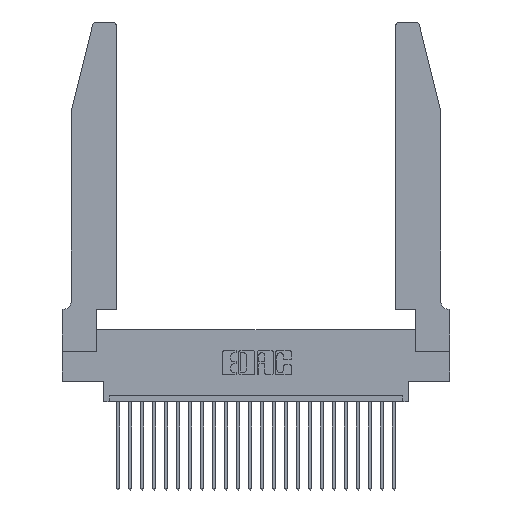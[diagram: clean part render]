
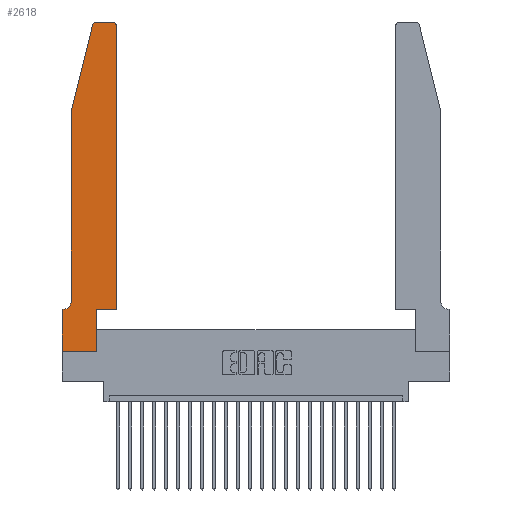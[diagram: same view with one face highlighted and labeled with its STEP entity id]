
A CAD part, top view. The second image highlights one B-rep face of the part: STEP entity #2618.
In plain terms, the highlighted planar face has unit normal (0, 0, 1).
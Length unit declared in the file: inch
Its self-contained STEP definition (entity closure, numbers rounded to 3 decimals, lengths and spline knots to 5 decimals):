
#230 = VERTEX_POINT ( 'NONE', #23160 ) ;
#433 = DIRECTION ( 'NONE',  ( 0., -1., 0. ) ) ;
#896 = EDGE_CURVE ( 'NONE', #230, #17937, #6956, .T. ) ;
#1086 = EDGE_CURVE ( 'NONE', #10948, #24289, #15489, .T. ) ;
#1366 = CIRCLE ( 'NONE', #4553, 0.03 ) ;
#1383 = ORIENTED_EDGE ( 'NONE', *, *, #7113, .T. ) ;
#1729 = EDGE_CURVE ( 'NONE', #17937, #22963, #1366, .T. ) ;
#1755 = LINE ( 'NONE', #19848, #10994 ) ;
#1852 = CARTESIAN_POINT ( 'NONE',  ( 0.4505, 0.35, 0.37 ) ) ;
#2592 = CARTESIAN_POINT ( 'NONE',  ( 0.4505, 0.35, 0.37 ) ) ;
#2618 = ADVANCED_FACE ( 'NONE', ( #6863 ), #22979, .T. ) ;
#2631 = VERTEX_POINT ( 'NONE', #15314 ) ;
#2958 = DIRECTION ( 'NONE',  ( 0., -1., 0. ) ) ;
#2971 = EDGE_CURVE ( 'NONE', #2631, #9389, #23330, .T. ) ;
#3082 = ORIENTED_EDGE ( 'NONE', *, *, #896, .T. ) ;
#3257 = VECTOR ( 'NONE', #22473, 39.37008 ) ;
#3511 = DIRECTION ( 'NONE',  ( 1., 0., 0. ) ) ;
#3547 = EDGE_CURVE ( 'NONE', #24289, #2631, #18083, .T. ) ;
#3821 = CARTESIAN_POINT ( 'NONE',  ( 0.284, 2.75, 0.37 ) ) ;
#3887 = CARTESIAN_POINT ( 'NONE',  ( 0., 0., 0.37 ) ) ;
#3987 = LINE ( 'NONE', #21486, #10465 ) ;
#4170 = EDGE_CURVE ( 'NONE', #19322, #5123, #21759, .T. ) ;
#4172 = LINE ( 'NONE', #19695, #13383 ) ;
#4553 = AXIS2_PLACEMENT_3D ( 'NONE', #25098, #15350, #10083 ) ;
#5013 = CARTESIAN_POINT ( 'NONE',  ( 0.4505, 2.72, 0.37 ) ) ;
#5123 = VERTEX_POINT ( 'NONE', #5013 ) ;
#6188 = VECTOR ( 'NONE', #14254, 39.37008 ) ;
#6364 = LINE ( 'NONE', #2592, #3257 ) ;
#6439 = ORIENTED_EDGE ( 'NONE', *, *, #19100, .T. ) ;
#6863 = FACE_OUTER_BOUND ( 'NONE', #10393, .T. ) ;
#6956 = LINE ( 'NONE', #8220, #20055 ) ;
#7113 = EDGE_CURVE ( 'NONE', #5123, #230, #16037, .T. ) ;
#7621 = DIRECTION ( 'NONE',  ( 0., 0., 1. ) ) ;
#7984 = ORIENTED_EDGE ( 'NONE', *, *, #4170, .T. ) ;
#8146 = CARTESIAN_POINT ( 'NONE',  ( 0.2865, 0., 0.37 ) ) ;
#8220 = CARTESIAN_POINT ( 'NONE',  ( 0.2605, 2.75, 0.37 ) ) ;
#8775 = CARTESIAN_POINT ( 'NONE',  ( 0.0055, 0.35, 0.37 ) ) ;
#9258 = LINE ( 'NONE', #21829, #19593 ) ;
#9281 = CARTESIAN_POINT ( 'NONE',  ( 0.4505, 0.35, 0.37 ) ) ;
#9389 = VERTEX_POINT ( 'NONE', #3887 ) ;
#9543 = CARTESIAN_POINT ( 'NONE',  ( 0., 0.35, 0.37 ) ) ;
#9842 = AXIS2_PLACEMENT_3D ( 'NONE', #9543, #7621, #21272 ) ;
#9856 = EDGE_CURVE ( 'NONE', #22963, #14524, #1755, .T. ) ;
#10039 = DIRECTION ( 'NONE',  ( 1., 0., 0. ) ) ;
#10083 = DIRECTION ( 'NONE',  ( 1., 0., 0. ) ) ;
#10370 = DIRECTION ( 'NONE',  ( 0., 1., 0. ) ) ;
#10393 = EDGE_LOOP ( 'NONE', ( #3082, #16094, #24740, #11400, #17698, #21245, #12485, #21521, #23491, #6439, #7984, #1383 ) ) ;
#10465 = VECTOR ( 'NONE', #10370, 39.37008 ) ;
#10948 = VERTEX_POINT ( 'NONE', #14444 ) ;
#10994 = VECTOR ( 'NONE', #12425, 39.37008 ) ;
#11400 = ORIENTED_EDGE ( 'NONE', *, *, #17654, .T. ) ;
#11937 = EDGE_CURVE ( 'NONE', #9389, #21149, #4172, .T. ) ;
#12398 = CARTESIAN_POINT ( 'NONE',  ( 0.25487, 2.72718, 0.37 ) ) ;
#12425 = DIRECTION ( 'NONE',  ( -0.239, -0.971, 0. ) ) ;
#12485 = ORIENTED_EDGE ( 'NONE', *, *, #2971, .T. ) ;
#12700 = DIRECTION ( 'NONE',  ( -1., 0., 0. ) ) ;
#13383 = VECTOR ( 'NONE', #10039, 39.37008 ) ;
#13565 = CARTESIAN_POINT ( 'NONE',  ( 0.4205, 2.72, 0.37 ) ) ;
#14254 = DIRECTION ( 'NONE',  ( -1., 0., 0. ) ) ;
#14444 = CARTESIAN_POINT ( 'NONE',  ( 0.0755, 0.42, 0.37 ) ) ;
#14524 = VERTEX_POINT ( 'NONE', #24292 ) ;
#15094 = VECTOR ( 'NONE', #2958, 39.37008 ) ;
#15314 = CARTESIAN_POINT ( 'NONE',  ( 0., 0.35, 0.37 ) ) ;
#15350 = DIRECTION ( 'NONE',  ( 0., 0., 1. ) ) ;
#15479 = CARTESIAN_POINT ( 'NONE',  ( 0.0055, 0.42, 0.37 ) ) ;
#15489 = CIRCLE ( 'NONE', #24383, 0.07 ) ;
#16037 = CIRCLE ( 'NONE', #16594, 0.03 ) ;
#16094 = ORIENTED_EDGE ( 'NONE', *, *, #1729, .T. ) ;
#16173 = VERTEX_POINT ( 'NONE', #18933 ) ;
#16594 = AXIS2_PLACEMENT_3D ( 'NONE', #13565, #25335, #3511 ) ;
#16916 = DIRECTION ( 'NONE',  ( -1., 0., 0. ) ) ;
#17654 = EDGE_CURVE ( 'NONE', #14524, #10948, #9258, .T. ) ;
#17698 = ORIENTED_EDGE ( 'NONE', *, *, #1086, .T. ) ;
#17937 = VERTEX_POINT ( 'NONE', #3821 ) ;
#18083 = LINE ( 'NONE', #18309, #6188 ) ;
#18309 = CARTESIAN_POINT ( 'NONE',  ( 0.0755, 0.35, 0.37 ) ) ;
#18924 = DIRECTION ( 'NONE',  ( 0., 0., -1. ) ) ;
#18933 = CARTESIAN_POINT ( 'NONE',  ( 0.2865, 0.35, 0.37 ) ) ;
#19100 = EDGE_CURVE ( 'NONE', #16173, #19322, #6364, .T. ) ;
#19322 = VERTEX_POINT ( 'NONE', #9281 ) ;
#19593 = VECTOR ( 'NONE', #433, 39.37008 ) ;
#19695 = CARTESIAN_POINT ( 'NONE',  ( 0., 0., 0.37 ) ) ;
#19848 = CARTESIAN_POINT ( 'NONE',  ( 0.0755, 2., 0.37 ) ) ;
#20055 = VECTOR ( 'NONE', #12700, 39.37008 ) ;
#21149 = VERTEX_POINT ( 'NONE', #8146 ) ;
#21151 = VECTOR ( 'NONE', #23378, 39.37008 ) ;
#21245 = ORIENTED_EDGE ( 'NONE', *, *, #3547, .T. ) ;
#21272 = DIRECTION ( 'NONE',  ( 1., 0., 0. ) ) ;
#21486 = CARTESIAN_POINT ( 'NONE',  ( 0.2865, 0.35, 0.37 ) ) ;
#21521 = ORIENTED_EDGE ( 'NONE', *, *, #11937, .T. ) ;
#21759 = LINE ( 'NONE', #1852, #21151 ) ;
#21829 = CARTESIAN_POINT ( 'NONE',  ( 0.0755, 2., 0.37 ) ) ;
#22473 = DIRECTION ( 'NONE',  ( 1., 0., 0. ) ) ;
#22963 = VERTEX_POINT ( 'NONE', #12398 ) ;
#22979 = PLANE ( 'NONE',  #9842 ) ;
#23160 = CARTESIAN_POINT ( 'NONE',  ( 0.4205, 2.75, 0.37 ) ) ;
#23330 = LINE ( 'NONE', #24445, #15094 ) ;
#23378 = DIRECTION ( 'NONE',  ( 0., 1., 0. ) ) ;
#23491 = ORIENTED_EDGE ( 'NONE', *, *, #25250, .T. ) ;
#24289 = VERTEX_POINT ( 'NONE', #8775 ) ;
#24292 = CARTESIAN_POINT ( 'NONE',  ( 0.0755, 2., 0.37 ) ) ;
#24383 = AXIS2_PLACEMENT_3D ( 'NONE', #15479, #18924, #16916 ) ;
#24445 = CARTESIAN_POINT ( 'NONE',  ( 0., 0., 0.37 ) ) ;
#24740 = ORIENTED_EDGE ( 'NONE', *, *, #9856, .T. ) ;
#25098 = CARTESIAN_POINT ( 'NONE',  ( 0.284, 2.72, 0.37 ) ) ;
#25250 = EDGE_CURVE ( 'NONE', #21149, #16173, #3987, .T. ) ;
#25335 = DIRECTION ( 'NONE',  ( 0., 0., 1. ) ) ;
